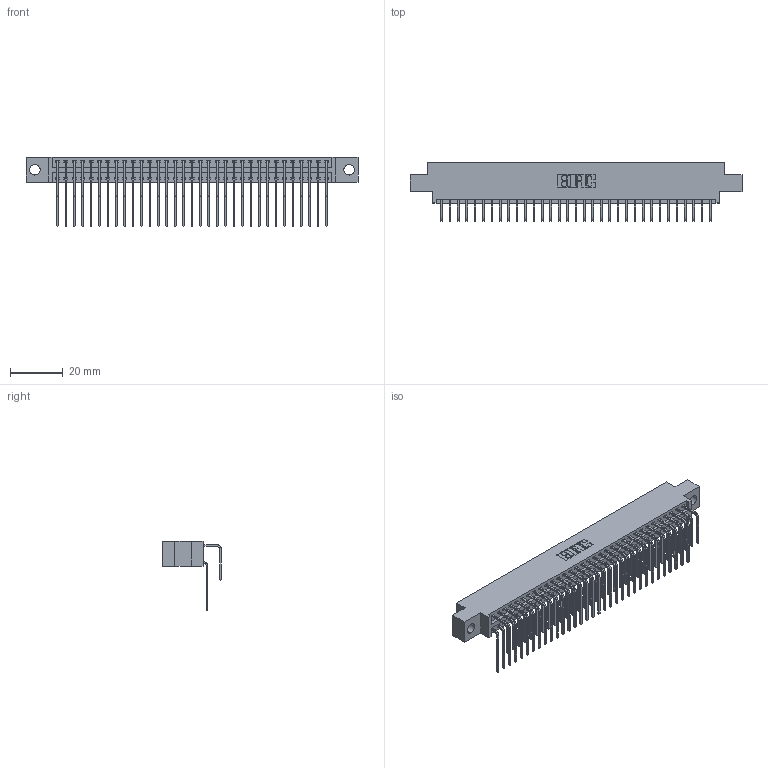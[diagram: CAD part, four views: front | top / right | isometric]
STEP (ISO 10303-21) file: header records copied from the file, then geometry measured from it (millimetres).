
FILE_DESCRIPTION (( 'STEP AP203' ), '1' );
FILE_NAME ('396-066-558-804.STEP', '2018-09-08T20:06:15', ( '' ), ( '' ), 'SwSTEP 2.0', 'SolidWorks 2016', '' );
FILE_SCHEMA (( 'CONFIG_CONTROL_DESIGN' ));
Length unit declared in the file: inch
Products named in the file (4): 345-292-001_558 Tail - 2; 396-066-558-804; 346 Part_0.170 Offset - 0.156 Dia-TH; 345-292-001_558 559 Tail - 1
Assembly tree (67 placements, depth 2):
  396-066-558-804
    346 Part_0.170 Offset - 0.156 Dia-TH
    345-292-001_558 559 Tail - 1  x33
    345-292-001_558 Tail - 2  x33
Bounding box: 125.35 x 22.16 x 26.16 mm (x, y, z)
Volume: 12291.4 mm3; surface area: 18573.5 mm2
Topology: 67 solids, 67 shells, 3690 faces, 10967 edges, 7222 vertices
Faces by surface type: plane 2522, cylinder 1168
Entity records: 24667 total; most frequent: CARTESIAN_POINT 4131, ORIENTED_EDGE 4014, DIRECTION 3663, EDGE_CURVE 2007, LINE 1703, VECTOR 1703, VERTEX_POINT 1334, AXIS2_PLACEMENT_3D 980
